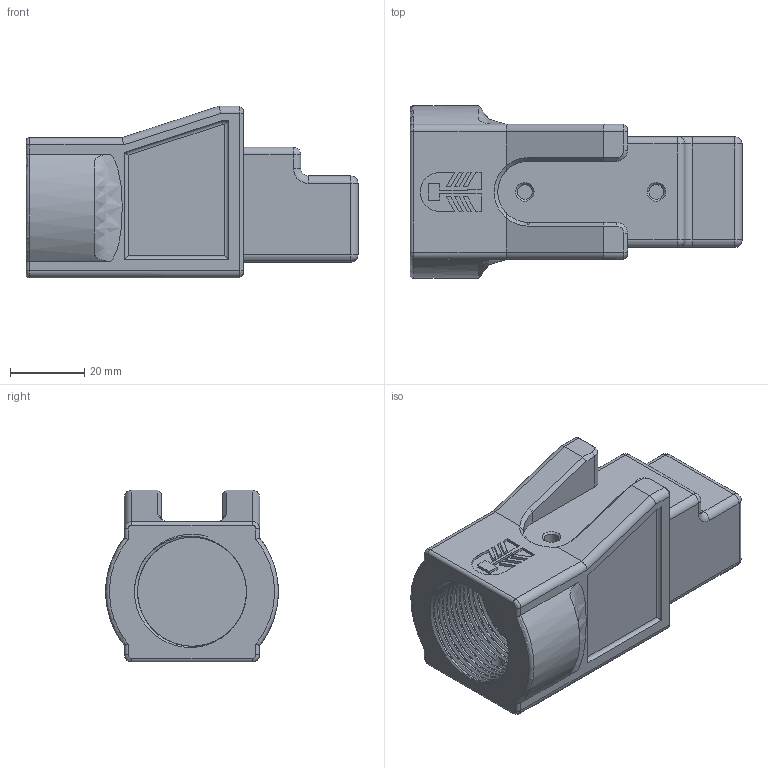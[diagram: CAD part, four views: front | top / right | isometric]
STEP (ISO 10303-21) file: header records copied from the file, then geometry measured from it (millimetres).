
FILE_DESCRIPTION(/* description */ (''),/* implementation_level */ '2;1');
FILE_NAME(/* name */ 'AK AR Stock Adapter v33.step',/* time_stamp */ '2022-04-15T18:51:23-05:00',/* author */ (''),/* organization */ (''),/* preprocessor_version */ 'ST-DEVELOPER v18.1',/* originating_system */ 'Autodesk Translation Framework v10.14.0.1471',/* authorisation */ '');
FILE_SCHEMA (('AUTOMOTIVE_DESIGN { 1 0 10303 214 3 1 1 }'));
Length unit declared in the file: millimetre
Products named in the file (1): AK AR Stock Adapter
Bounding box: 89.61 x 46.63 x 46.41 mm (x, y, z)
Volume: 96073 mm3; surface area: 19275 mm2
Topology: 1 solids, 1 shells, 184 faces, 481 edges, 303 vertices
Faces by surface type: plane 75, cylinder 74, bspline 16, cone 9, sphere 6, torus 4
Full cylindrical faces by diameter (mm): 3.605 x1, 4 x2, 29.411 x8, 31.067 x9
Entity records: 9102 total; most frequent: CARTESIAN_POINT 4728, ORIENTED_EDGE 960, DIRECTION 813, EDGE_CURVE 480, VERTEX_POINT 303, LINE 283, VECTOR 283, AXIS2_PLACEMENT_3D 265
